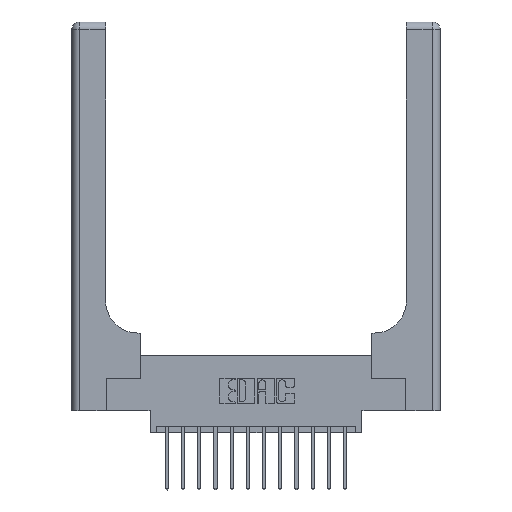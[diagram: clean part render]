
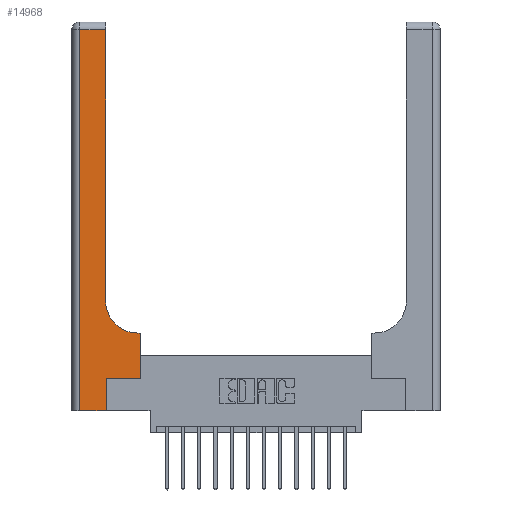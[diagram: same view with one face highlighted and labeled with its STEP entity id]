
A CAD part, top view. The second image highlights one B-rep face of the part: STEP entity #14968.
In plain terms, the highlighted planar face has unit normal (0, 0, 1).
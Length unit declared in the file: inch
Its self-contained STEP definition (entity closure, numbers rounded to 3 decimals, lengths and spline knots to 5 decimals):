
#158 = LINE ( 'NONE', #9136, #17005 ) ;
#216 = CARTESIAN_POINT ( 'NONE',  ( 0.528, 0.25, 0.37 ) ) ;
#299 = VERTEX_POINT ( 'NONE', #12605 ) ;
#306 = LINE ( 'NONE', #4324, #6988 ) ;
#795 = VERTEX_POINT ( 'NONE', #1546 ) ;
#806 = CARTESIAN_POINT ( 'NONE',  ( 0.265, 0., 0.37 ) ) ;
#1046 = CARTESIAN_POINT ( 'NONE',  ( 0.06, 0., 0.37 ) ) ;
#1338 = ORIENTED_EDGE ( 'NONE', *, *, #12561, .T. ) ;
#1546 = CARTESIAN_POINT ( 'NONE',  ( 0.265, 0.25, 0.37 ) ) ;
#1749 = LINE ( 'NONE', #9949, #8417 ) ;
#1791 = ORIENTED_EDGE ( 'NONE', *, *, #6749, .T. ) ;
#2166 = CARTESIAN_POINT ( 'NONE',  ( 0.51, 0.6, 0.37 ) ) ;
#2498 = DIRECTION ( 'NONE',  ( 1., 0., 0. ) ) ;
#2610 = EDGE_CURVE ( 'NONE', #3326, #299, #306, .T. ) ;
#3140 = VERTEX_POINT ( 'NONE', #8160 ) ;
#3273 = CARTESIAN_POINT ( 'NONE',  ( 0.51, 0.85, 0.37 ) ) ;
#3326 = VERTEX_POINT ( 'NONE', #9718 ) ;
#3655 = PLANE ( 'NONE',  #14440 ) ;
#3671 = ORIENTED_EDGE ( 'NONE', *, *, #6943, .T. ) ;
#4131 = LINE ( 'NONE', #5212, #6859 ) ;
#4324 = CARTESIAN_POINT ( 'NONE',  ( 0., 2.94, 0.37 ) ) ;
#4596 = VECTOR ( 'NONE', #6097, 39.37008 ) ;
#4604 = DIRECTION ( 'NONE',  ( 1., 0., 0. ) ) ;
#4788 = CARTESIAN_POINT ( 'NONE',  ( 0.06, 3., 0.37 ) ) ;
#4877 = LINE ( 'NONE', #6053, #11536 ) ;
#4997 = DIRECTION ( 'NONE',  ( 0., 0., -1. ) ) ;
#5068 = VERTEX_POINT ( 'NONE', #806 ) ;
#5110 = VERTEX_POINT ( 'NONE', #6235 ) ;
#5212 = CARTESIAN_POINT ( 'NONE',  ( 0.26, 3., 0.37 ) ) ;
#5793 = FACE_OUTER_BOUND ( 'NONE', #8834, .T. ) ;
#6053 = CARTESIAN_POINT ( 'NONE',  ( 0.265, 0.25, 0.37 ) ) ;
#6097 = DIRECTION ( 'NONE',  ( 0., 1., 0. ) ) ;
#6235 = CARTESIAN_POINT ( 'NONE',  ( 0.528, 0.6, 0.37 ) ) ;
#6749 = EDGE_CURVE ( 'NONE', #14695, #5110, #1749, .T. ) ;
#6778 = EDGE_CURVE ( 'NONE', #795, #14695, #4877, .T. ) ;
#6859 = VECTOR ( 'NONE', #10776, 39.37008 ) ;
#6943 = EDGE_CURVE ( 'NONE', #5110, #9731, #16085, .T. ) ;
#6988 = VECTOR ( 'NONE', #16284, 39.37008 ) ;
#7733 = LINE ( 'NONE', #10097, #4596 ) ;
#7750 = ORIENTED_EDGE ( 'NONE', *, *, #2610, .T. ) ;
#7912 = LINE ( 'NONE', #4788, #14128 ) ;
#8160 = CARTESIAN_POINT ( 'NONE',  ( 0.26, 0.85, 0.37 ) ) ;
#8217 = CIRCLE ( 'NONE', #15531, 0.25 ) ;
#8417 = VECTOR ( 'NONE', #16544, 39.37008 ) ;
#8834 = EDGE_LOOP ( 'NONE', ( #10373, #7750, #12964, #11541, #1338, #16756, #1791, #3671, #15360 ) ) ;
#9028 = VECTOR ( 'NONE', #11849, 39.37008 ) ;
#9136 = CARTESIAN_POINT ( 'NONE',  ( 0., 0., 0.37 ) ) ;
#9642 = EDGE_CURVE ( 'NONE', #299, #13254, #7912, .T. ) ;
#9718 = CARTESIAN_POINT ( 'NONE',  ( 0.26, 2.94, 0.37 ) ) ;
#9731 = VERTEX_POINT ( 'NONE', #2166 ) ;
#9949 = CARTESIAN_POINT ( 'NONE',  ( 0.528, 0.25, 0.37 ) ) ;
#10097 = CARTESIAN_POINT ( 'NONE',  ( 0.265, 0., 0.37 ) ) ;
#10373 = ORIENTED_EDGE ( 'NONE', *, *, #14155, .T. ) ;
#10386 = EDGE_CURVE ( 'NONE', #13254, #5068, #158, .T. ) ;
#10534 = CARTESIAN_POINT ( 'NONE',  ( 0.26, 0.6, 0.37 ) ) ;
#10776 = DIRECTION ( 'NONE',  ( 0., 1., 0. ) ) ;
#11536 = VECTOR ( 'NONE', #15332, 39.37008 ) ;
#11541 = ORIENTED_EDGE ( 'NONE', *, *, #10386, .T. ) ;
#11849 = DIRECTION ( 'NONE',  ( -1., 0., 0. ) ) ;
#12561 = EDGE_CURVE ( 'NONE', #5068, #795, #7733, .T. ) ;
#12569 = DIRECTION ( 'NONE',  ( 0., 0., -1. ) ) ;
#12605 = CARTESIAN_POINT ( 'NONE',  ( 0.06, 2.94, 0.37 ) ) ;
#12950 = CARTESIAN_POINT ( 'NONE',  ( 0., 3., 0.37 ) ) ;
#12964 = ORIENTED_EDGE ( 'NONE', *, *, #9642, .T. ) ;
#13254 = VERTEX_POINT ( 'NONE', #1046 ) ;
#14080 = DIRECTION ( 'NONE',  ( 0., -1., 0. ) ) ;
#14128 = VECTOR ( 'NONE', #14080, 39.37008 ) ;
#14155 = EDGE_CURVE ( 'NONE', #3140, #3326, #4131, .T. ) ;
#14289 = DIRECTION ( 'NONE',  ( -1., 0., 0. ) ) ;
#14440 = AXIS2_PLACEMENT_3D ( 'NONE', #12950, #4997, #14289 ) ;
#14695 = VERTEX_POINT ( 'NONE', #216 ) ;
#14968 = ADVANCED_FACE ( 'NONE', ( #5793 ), #3655, .F. ) ;
#15332 = DIRECTION ( 'NONE',  ( 1., 0., 0. ) ) ;
#15360 = ORIENTED_EDGE ( 'NONE', *, *, #16646, .T. ) ;
#15531 = AXIS2_PLACEMENT_3D ( 'NONE', #3273, #12569, #4604 ) ;
#16085 = LINE ( 'NONE', #10534, #9028 ) ;
#16284 = DIRECTION ( 'NONE',  ( -1., 0., 0. ) ) ;
#16544 = DIRECTION ( 'NONE',  ( 0., 1., 0. ) ) ;
#16646 = EDGE_CURVE ( 'NONE', #9731, #3140, #8217, .T. ) ;
#16756 = ORIENTED_EDGE ( 'NONE', *, *, #6778, .T. ) ;
#17005 = VECTOR ( 'NONE', #2498, 39.37008 ) ;
